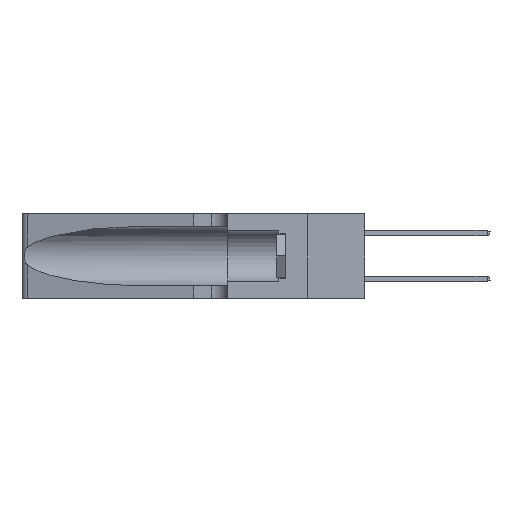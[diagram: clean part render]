
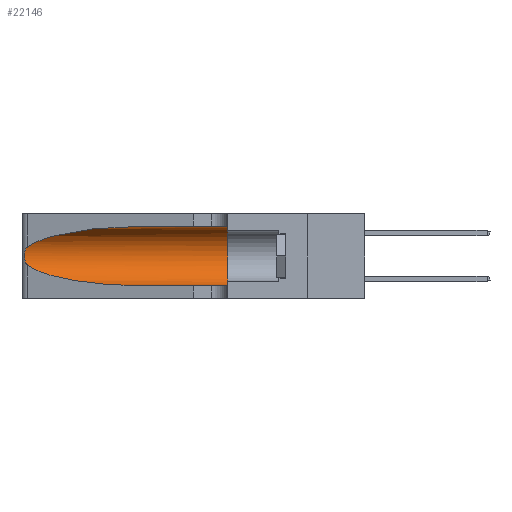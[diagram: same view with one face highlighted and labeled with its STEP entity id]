
A CAD part, left-side view. The second image highlights one B-rep face of the part: STEP entity #22146.
In plain terms, the highlighted cylindrical face has radius 3.308 mm (diameter 6.617 mm), a partial arc.
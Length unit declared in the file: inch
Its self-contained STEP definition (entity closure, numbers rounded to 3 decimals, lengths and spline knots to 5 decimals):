
#202 = AXIS2_PLACEMENT_3D ( 'NONE', #2513, #28391, #6268 ) ;
#222 = CARTESIAN_POINT ( 'NONE',  ( 0.1305, 0.72297, 0.31525 ) ) ;
#1801 = VERTEX_POINT ( 'NONE', #23762 ) ;
#1971 = CARTESIAN_POINT ( 'NONE',  ( 0.25555, 1.22993, 0.14849 ) ) ;
#2513 = CARTESIAN_POINT ( 'NONE',  ( 0.1305, 1.61858, 0.185 ) ) ;
#3965 = ORIENTED_EDGE ( 'NONE', *, *, #19081, .T. ) ;
#4044 = DIRECTION ( 'NONE',  ( 0., -1., 0. ) ) ;
#6268 = DIRECTION ( 'NONE',  ( 0., 0., -1. ) ) ;
#7734 = EDGE_CURVE ( 'NONE', #44043, #16677, #7796, .T. ) ;
#7750 = CARTESIAN_POINT ( 'NONE',  ( 0.25487, 1.22718, 0.22369 ) ) ;
#7796 = CIRCLE ( 'NONE', #12419, 0.13025 ) ;
#9323 = CARTESIAN_POINT ( 'NONE',  ( 0.25787, 1.23484, 0.2124 ) ) ;
#9868 = B_SPLINE_CURVE_WITH_KNOTS ( 'NONE', 3,
 ( #27713, #45742, #31360, #9323, #34978, #13109, #38588, #16857, #42224, #20575, #45901, #24213, #1971, #27858 ),
 .UNSPECIFIED., .F., .F.,
 ( 4, 2, 2, 2, 2, 2, 4 ),
 ( 0., 0.00027, 0.00053, 0.00107, 0.0016, 0.00187, 0.00214 ),
 .UNSPECIFIED. ) ;
#10225 = ORIENTED_EDGE ( 'NONE', *, *, #7734, .F. ) ;
#12419 = AXIS2_PLACEMENT_3D ( 'NONE', #15523, #40891, #19247 ) ;
#13109 = CARTESIAN_POINT ( 'NONE',  ( 0.26018, 1.23835, 0.19895 ) ) ;
#13288 = VERTEX_POINT ( 'NONE', #17816 ) ;
#15523 = CARTESIAN_POINT ( 'NONE',  ( 0.1305, 0.35, 0.185 ) ) ;
#16677 = VERTEX_POINT ( 'NONE', #38956 ) ;
#16857 = CARTESIAN_POINT ( 'NONE',  ( 0.26075, 1.23896, 0.178 ) ) ;
#17423 = VECTOR ( 'NONE', #4044, 39.37008 ) ;
#17631 = CARTESIAN_POINT ( 'NONE',  ( 0.25487, 1.22718, 0.22369 ) ) ;
#17816 = CARTESIAN_POINT ( 'NONE',  ( 0.25487, 1.22718, 0.14631 ) ) ;
#18353 = CARTESIAN_POINT ( 'NONE',  ( 0.1305, 0.72297, 0.05475 ) ) ;
#18914 = CARTESIAN_POINT ( 'NONE',  ( 0.1305, 1.61858, 0.05475 ) ) ;
#19081 = EDGE_CURVE ( 'NONE', #47188, #13288, #9868, .T. ) ;
#19247 = DIRECTION ( 'NONE',  ( 0., 0., 1. ) ) ;
#19686 = LINE ( 'NONE', #21292, #37775 ) ;
#20575 = CARTESIAN_POINT ( 'NONE',  ( 0.25856, 1.23593, 0.16098 ) ) ;
#21292 = CARTESIAN_POINT ( 'NONE',  ( 0.1305, 1.61858, 0.31525 ) ) ;
#21360 = ORIENTED_EDGE ( 'NONE', *, *, #30685, .F. ) ;
#22146 = ADVANCED_FACE ( 'NONE', ( #44494 ), #25228, .F. ) ;
#22238 = CARTESIAN_POINT ( 'NONE',  ( 0.1305, 0.72297, 0.31525 ) ) ;
#22553 = CARTESIAN_POINT ( 'NONE',  ( 0.18966, 0.96281, 0.31525 ) ) ;
#23458 = ORIENTED_EDGE ( 'NONE', *, *, #37389, .T. ) ;
#23762 = CARTESIAN_POINT ( 'NONE',  ( 0.1305, 0.72297, 0.05475 ) ) ;
#24213 = CARTESIAN_POINT ( 'NONE',  ( 0.25639, 1.23186, 0.15144 ) ) ;
#24921 = DIRECTION ( 'NONE',  ( 0., -1., 0. ) ) ;
#25228 = CYLINDRICAL_SURFACE ( 'NONE', #202, 0.13025 ) ;
#25384 = EDGE_CURVE ( 'NONE', #34402, #47188, #31964, .T. ) ;
#25522 = CARTESIAN_POINT ( 'NONE',  ( 0.25487, 1.22718, 0.14631 ) ) ;
#27140 = LINE ( 'NONE', #18914, #17423 ) ;
#27713 = CARTESIAN_POINT ( 'NONE',  ( 0.25487, 1.22718, 0.22369 ) ) ;
#27858 = CARTESIAN_POINT ( 'NONE',  ( 0.25487, 1.22718, 0.14631 ) ) ;
#28391 = DIRECTION ( 'NONE',  ( 0., -1., 0. ) ) ;
#29838 = CARTESIAN_POINT ( 'NONE',  ( 0.2373, 1.15595, 0.28018 ) ) ;
#30685 = EDGE_CURVE ( 'NONE', #34402, #44043, #19686, .T. ) ;
#31360 = CARTESIAN_POINT ( 'NONE',  ( 0.25639, 1.23184, 0.21858 ) ) ;
#31964 =( BOUNDED_CURVE ( )  B_SPLINE_CURVE ( 3, ( #222, #22553, #29838, #7750 ),
 .UNSPECIFIED., .F., .T. ) 
 B_SPLINE_CURVE_WITH_KNOTS ( ( 4, 4 ),
 ( 1.5708, 2.84003 ),
 .UNSPECIFIED. ) 
 CURVE ( )  GEOMETRIC_REPRESENTATION_ITEM ( )  RATIONAL_B_SPLINE_CURVE ( ( 1., 0.87, 0.87, 1. ) ) 
 REPRESENTATION_ITEM ( '' )  );
#32161 = ORIENTED_EDGE ( 'NONE', *, *, #25384, .T. ) ;
#32624 = EDGE_LOOP ( 'NONE', ( #32161, #3965, #41834, #23458, #10225, #21360 ) ) ;
#34402 = VERTEX_POINT ( 'NONE', #22238 ) ;
#34978 = CARTESIAN_POINT ( 'NONE',  ( 0.25854, 1.2359, 0.20912 ) ) ;
#36850 =( BOUNDED_CURVE ( )  B_SPLINE_CURVE ( 3, ( #25522, #43537, #40047, #18353 ),
 .UNSPECIFIED., .F., .F. ) 
 B_SPLINE_CURVE_WITH_KNOTS ( ( 4, 4 ),
 ( 3.44316, 4.71239 ),
 .UNSPECIFIED. ) 
 CURVE ( )  GEOMETRIC_REPRESENTATION_ITEM ( )  RATIONAL_B_SPLINE_CURVE ( ( 1., 0.87, 0.87, 1. ) ) 
 REPRESENTATION_ITEM ( '' )  );
#37389 = EDGE_CURVE ( 'NONE', #1801, #16677, #27140, .T. ) ;
#37775 = VECTOR ( 'NONE', #24921, 39.37008 ) ;
#38588 = CARTESIAN_POINT ( 'NONE',  ( 0.26075, 1.23896, 0.19203 ) ) ;
#38956 = CARTESIAN_POINT ( 'NONE',  ( 0.1305, 0.35, 0.05475 ) ) ;
#40047 = CARTESIAN_POINT ( 'NONE',  ( 0.18966, 0.96281, 0.05475 ) ) ;
#40891 = DIRECTION ( 'NONE',  ( 0., 1., 0. ) ) ;
#41834 = ORIENTED_EDGE ( 'NONE', *, *, #42480, .T. ) ;
#42224 = CARTESIAN_POINT ( 'NONE',  ( 0.26017, 1.23833, 0.17102 ) ) ;
#42480 = EDGE_CURVE ( 'NONE', #13288, #1801, #36850, .T. ) ;
#43110 = CARTESIAN_POINT ( 'NONE',  ( 0.1305, 0.35, 0.31525 ) ) ;
#43537 = CARTESIAN_POINT ( 'NONE',  ( 0.2373, 1.15595, 0.08982 ) ) ;
#44043 = VERTEX_POINT ( 'NONE', #43110 ) ;
#44494 = FACE_OUTER_BOUND ( 'NONE', #32624, .T. ) ;
#45742 = CARTESIAN_POINT ( 'NONE',  ( 0.25555, 1.22994, 0.2215 ) ) ;
#45901 = CARTESIAN_POINT ( 'NONE',  ( 0.25789, 1.23486, 0.15765 ) ) ;
#47188 = VERTEX_POINT ( 'NONE', #17631 ) ;
